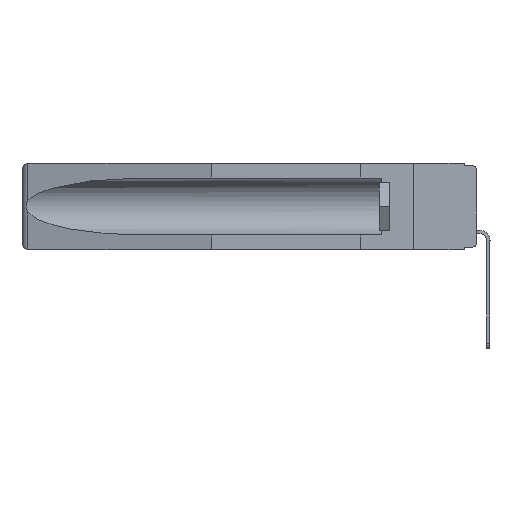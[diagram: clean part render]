
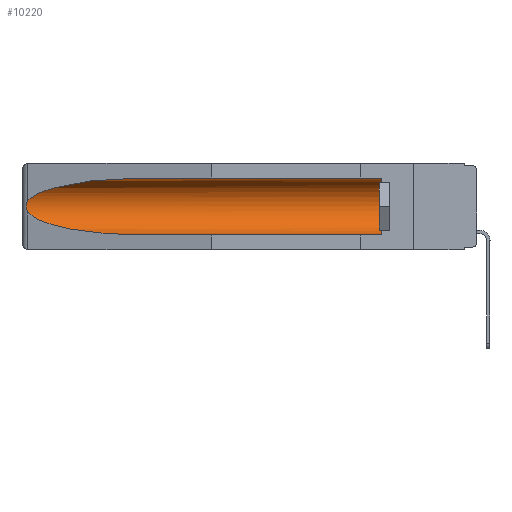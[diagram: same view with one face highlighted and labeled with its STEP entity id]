
A CAD part, left-side view. The second image highlights one B-rep face of the part: STEP entity #10220.
In plain terms, the highlighted cylindrical face has radius 2.857 mm (diameter 5.715 mm), a partial arc.
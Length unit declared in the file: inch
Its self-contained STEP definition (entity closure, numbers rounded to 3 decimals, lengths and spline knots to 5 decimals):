
#479 = CIRCLE ( 'NONE', #7765, 0.1125 ) ;
#799 = ORIENTED_EDGE ( 'NONE', *, *, #12659, .T. ) ;
#1174 = CARTESIAN_POINT ( 'NONE',  ( 0.26537, 1.52718, -0.14972 ) ) ;
#1431 = ORIENTED_EDGE ( 'NONE', *, *, #6779, .F. ) ;
#1459 = ORIENTED_EDGE ( 'NONE', *, *, #11078, .T. ) ;
#1661 = B_SPLINE_CURVE_WITH_KNOTS ( 'NONE', 3,
 ( #1174, #7828, #6632, #2370, #9451, #3821, #2190, #16410, #10826, #3730 ),
 .UNSPECIFIED., .F., .F.,
 ( 4, 2, 2, 2, 4 ),
 ( 0., 0.00029, 0.00058, 0.00087, 0.00117 ),
 .UNSPECIFIED. ) ;
#1915 = CARTESIAN_POINT ( 'NONE',  ( 0.155, 1.07973, -0.059 ) ) ;
#1987 = CARTESIAN_POINT ( 'NONE',  ( 0.155, -0.30754, -0.1715 ) ) ;
#2010 = CARTESIAN_POINT ( 'NONE',  ( 0.155, 0.126, -0.284 ) ) ;
#2190 = CARTESIAN_POINT ( 'NONE',  ( 0.2673, 1.53269, -0.17917 ) ) ;
#2370 = CARTESIAN_POINT ( 'NONE',  ( 0.2673, 1.5327, -0.16383 ) ) ;
#2564 = LINE ( 'NONE', #13865, #4295 ) ;
#3730 = CARTESIAN_POINT ( 'NONE',  ( 0.26537, 1.52718, -0.19328 ) ) ;
#3821 = CARTESIAN_POINT ( 'NONE',  ( 0.2675, 1.53308, -0.17534 ) ) ;
#3936 = EDGE_CURVE ( 'NONE', #14846, #13270, #17650, .T. ) ;
#4295 = VECTOR ( 'NONE', #12676, 39.37008 ) ;
#4329 = CARTESIAN_POINT ( 'NONE',  ( 0.155, 1.07973, -0.284 ) ) ;
#4727 = CARTESIAN_POINT ( 'NONE',  ( 0.155, 1.07973, -0.059 ) ) ;
#5097 = CARTESIAN_POINT ( 'NONE',  ( 0.25451, 1.48313, -0.09465 ) ) ;
#5178 = ORIENTED_EDGE ( 'NONE', *, *, #10631, .T. ) ;
#6513 = VECTOR ( 'NONE', #11789, 39.37008 ) ;
#6632 = CARTESIAN_POINT ( 'NONE',  ( 0.26654, 1.53092, -0.15636 ) ) ;
#6733 = ORIENTED_EDGE ( 'NONE', *, *, #3936, .T. ) ;
#6769 = CARTESIAN_POINT ( 'NONE',  ( 0.155, 0.126, -0.1715 ) ) ;
#6779 = EDGE_CURVE ( 'NONE', #9597, #18016, #14333, .T. ) ;
#6842 = AXIS2_PLACEMENT_3D ( 'NONE', #1987, #10262, #14279 ) ;
#7399 = CARTESIAN_POINT ( 'NONE',  ( 0.155, 1.07973, -0.284 ) ) ;
#7674 = ORIENTED_EDGE ( 'NONE', *, *, #17541, .T. ) ;
#7686 = CARTESIAN_POINT ( 'NONE',  ( 0.155, -0.30754, -0.284 ) ) ;
#7765 = AXIS2_PLACEMENT_3D ( 'NONE', #6769, #17917, #10957 ) ;
#7828 = CARTESIAN_POINT ( 'NONE',  ( 0.26597, 1.52961, -0.15275 ) ) ;
#8290 = FACE_OUTER_BOUND ( 'NONE', #15033, .T. ) ;
#8511 = CARTESIAN_POINT ( 'NONE',  ( 0.25451, 1.48313, -0.24835 ) ) ;
#9372 = VERTEX_POINT ( 'NONE', #10048 ) ;
#9451 = CARTESIAN_POINT ( 'NONE',  ( 0.2675, 1.53308, -0.16763 ) ) ;
#9477 = CYLINDRICAL_SURFACE ( 'NONE', #6842, 0.1125 ) ;
#9597 = VERTEX_POINT ( 'NONE', #2010 ) ;
#9969 = CARTESIAN_POINT ( 'NONE',  ( 0.21114, 1.30732, -0.284 ) ) ;
#10048 = CARTESIAN_POINT ( 'NONE',  ( 0.155, 0.126, -0.059 ) ) ;
#10220 = ADVANCED_FACE ( 'NONE', ( #8290 ), #9477, .F. ) ;
#10262 = DIRECTION ( 'NONE',  ( 0., 1., 0. ) ) ;
#10631 = EDGE_CURVE ( 'NONE', #17039, #18016, #11339, .T. ) ;
#10826 = CARTESIAN_POINT ( 'NONE',  ( 0.26597, 1.5296, -0.19026 ) ) ;
#10957 = DIRECTION ( 'NONE',  ( 0., 0., 1. ) ) ;
#11078 = EDGE_CURVE ( 'NONE', #9597, #9372, #479, .T. ) ;
#11339 =( BOUNDED_CURVE ( )  B_SPLINE_CURVE ( 3, ( #15359, #8511, #9969, #4329 ),
 .UNSPECIFIED., .F., .F. ) 
 B_SPLINE_CURVE_WITH_KNOTS ( ( 4, 4 ),
 ( 0.1948, 1.5708 ),
 .UNSPECIFIED. ) 
 CURVE ( )  GEOMETRIC_REPRESENTATION_ITEM ( )  RATIONAL_B_SPLINE_CURVE ( ( 1., 0.848, 0.848, 1. ) ) 
 REPRESENTATION_ITEM ( '' )  );
#11789 = DIRECTION ( 'NONE',  ( 0., 1., 0. ) ) ;
#12659 = EDGE_CURVE ( 'NONE', #9372, #14846, #2564, .T. ) ;
#12676 = DIRECTION ( 'NONE',  ( 0., 1., 0. ) ) ;
#13270 = VERTEX_POINT ( 'NONE', #15847 ) ;
#13865 = CARTESIAN_POINT ( 'NONE',  ( 0.155, -0.30754, -0.059 ) ) ;
#14279 = DIRECTION ( 'NONE',  ( 0., 0., 1. ) ) ;
#14333 = LINE ( 'NONE', #7686, #6513 ) ;
#14525 = CARTESIAN_POINT ( 'NONE',  ( 0.26537, 1.52718, -0.19328 ) ) ;
#14841 = CARTESIAN_POINT ( 'NONE',  ( 0.26537, 1.52718, -0.14972 ) ) ;
#14846 = VERTEX_POINT ( 'NONE', #1915 ) ;
#15033 = EDGE_LOOP ( 'NONE', ( #6733, #7674, #5178, #1431, #1459, #799 ) ) ;
#15359 = CARTESIAN_POINT ( 'NONE',  ( 0.26537, 1.52718, -0.19328 ) ) ;
#15847 = CARTESIAN_POINT ( 'NONE',  ( 0.26537, 1.52718, -0.14972 ) ) ;
#15857 = CARTESIAN_POINT ( 'NONE',  ( 0.21114, 1.30732, -0.059 ) ) ;
#16410 = CARTESIAN_POINT ( 'NONE',  ( 0.26655, 1.53094, -0.18657 ) ) ;
#17039 = VERTEX_POINT ( 'NONE', #14525 ) ;
#17541 = EDGE_CURVE ( 'NONE', #13270, #17039, #1661, .T. ) ;
#17650 =( BOUNDED_CURVE ( )  B_SPLINE_CURVE ( 3, ( #4727, #15857, #5097, #14841 ),
 .UNSPECIFIED., .F., .F. ) 
 B_SPLINE_CURVE_WITH_KNOTS ( ( 4, 4 ),
 ( 4.71239, 6.08839 ),
 .UNSPECIFIED. ) 
 CURVE ( )  GEOMETRIC_REPRESENTATION_ITEM ( )  RATIONAL_B_SPLINE_CURVE ( ( 1., 0.848, 0.848, 1. ) ) 
 REPRESENTATION_ITEM ( '' )  );
#17917 = DIRECTION ( 'NONE',  ( 0., -1., 0. ) ) ;
#18016 = VERTEX_POINT ( 'NONE', #7399 ) ;
